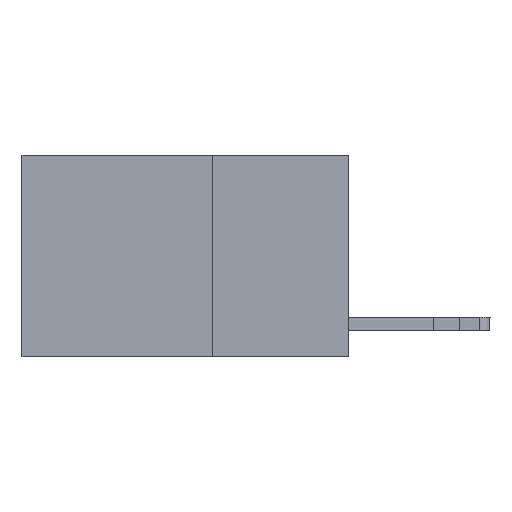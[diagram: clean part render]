
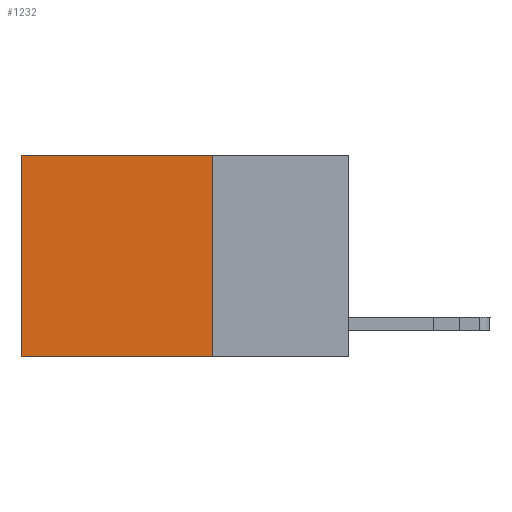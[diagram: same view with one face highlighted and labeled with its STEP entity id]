
A CAD part, left-side view. The second image highlights one B-rep face of the part: STEP entity #1232.
In plain terms, the highlighted planar face has unit normal (-1, 0, 0).
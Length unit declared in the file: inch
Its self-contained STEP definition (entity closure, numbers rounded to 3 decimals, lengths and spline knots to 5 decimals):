
#60 = DIRECTION ( 'NONE',  ( 1., 0., 0. ) ) ;
#1232 = ADVANCED_FACE ( 'NONE', ( #15187 ), #8809, .F. ) ;
#1441 = VERTEX_POINT ( 'NONE', #12208 ) ;
#1458 = CARTESIAN_POINT ( 'NONE',  ( 0.2625, 0.25, 0. ) ) ;
#1600 = EDGE_CURVE ( 'NONE', #4965, #3658, #1914, .T. ) ;
#1914 = LINE ( 'NONE', #3685, #13112 ) ;
#2101 = ORIENTED_EDGE ( 'NONE', *, *, #15857, .F. ) ;
#2196 = CARTESIAN_POINT ( 'NONE',  ( 0.2625, 0.25, 0. ) ) ;
#2626 = EDGE_LOOP ( 'NONE', ( #15994, #2101, #14259, #17496 ) ) ;
#3658 = VERTEX_POINT ( 'NONE', #14361 ) ;
#3685 = CARTESIAN_POINT ( 'NONE',  ( 0.2625, 0.25, 0. ) ) ;
#4965 = VERTEX_POINT ( 'NONE', #13091 ) ;
#6894 = VECTOR ( 'NONE', #13901, 39.37008 ) ;
#7260 = CARTESIAN_POINT ( 'NONE',  ( 0.2625, 0.6, 0. ) ) ;
#7306 = EDGE_CURVE ( 'NONE', #13677, #1441, #15153, .T. ) ;
#7673 = EDGE_CURVE ( 'NONE', #4965, #13677, #15134, .T. ) ;
#8809 = PLANE ( 'NONE',  #18468 ) ;
#10270 = DIRECTION ( 'NONE',  ( 0., 0., -1. ) ) ;
#11679 = DIRECTION ( 'NONE',  ( 0., 0., -1. ) ) ;
#12208 = CARTESIAN_POINT ( 'NONE',  ( 0.2625, 0.6, -0.37 ) ) ;
#13091 = CARTESIAN_POINT ( 'NONE',  ( 0.2625, 0.25, 0. ) ) ;
#13112 = VECTOR ( 'NONE', #16834, 39.37008 ) ;
#13677 = VERTEX_POINT ( 'NONE', #17537 ) ;
#13901 = DIRECTION ( 'NONE',  ( 0., 1., 0. ) ) ;
#14045 = VECTOR ( 'NONE', #18246, 39.37008 ) ;
#14259 = ORIENTED_EDGE ( 'NONE', *, *, #1600, .F. ) ;
#14361 = CARTESIAN_POINT ( 'NONE',  ( 0.2625, 0.25, -0.37 ) ) ;
#15134 = LINE ( 'NONE', #2196, #6894 ) ;
#15153 = LINE ( 'NONE', #7260, #18578 ) ;
#15187 = FACE_OUTER_BOUND ( 'NONE', #2626, .T. ) ;
#15857 = EDGE_CURVE ( 'NONE', #3658, #1441, #17928, .T. ) ;
#15994 = ORIENTED_EDGE ( 'NONE', *, *, #7306, .T. ) ;
#16758 = CARTESIAN_POINT ( 'NONE',  ( 0.2625, 0.25, -0.37 ) ) ;
#16834 = DIRECTION ( 'NONE',  ( 0., 0., -1. ) ) ;
#17496 = ORIENTED_EDGE ( 'NONE', *, *, #7673, .T. ) ;
#17537 = CARTESIAN_POINT ( 'NONE',  ( 0.2625, 0.6, 0. ) ) ;
#17928 = LINE ( 'NONE', #16758, #14045 ) ;
#18246 = DIRECTION ( 'NONE',  ( 0., 1., 0. ) ) ;
#18468 = AXIS2_PLACEMENT_3D ( 'NONE', #1458, #60, #10270 ) ;
#18578 = VECTOR ( 'NONE', #11679, 39.37008 ) ;
